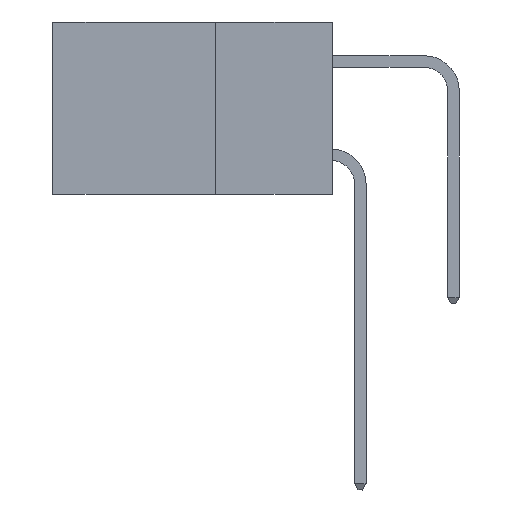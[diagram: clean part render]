
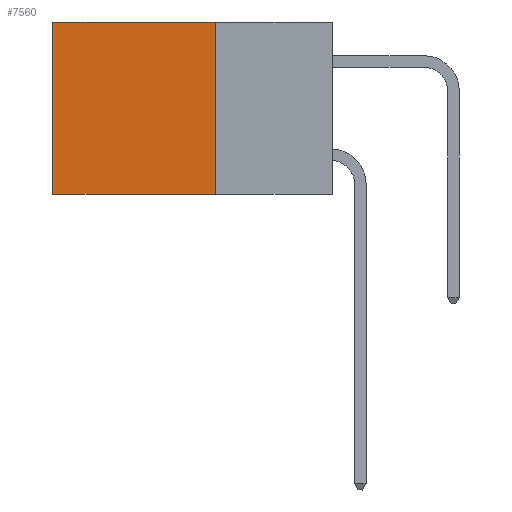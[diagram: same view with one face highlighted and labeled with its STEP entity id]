
A CAD part, left-side view. The second image highlights one B-rep face of the part: STEP entity #7560.
In plain terms, the highlighted planar face has unit normal (-1, 0, 0).
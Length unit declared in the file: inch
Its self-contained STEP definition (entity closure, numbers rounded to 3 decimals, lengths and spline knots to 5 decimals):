
#1771 = CARTESIAN_POINT ( 'NONE',  ( 0.298, 0.6, -0.37 ) ) ;
#1935 = VERTEX_POINT ( 'NONE', #1771 ) ;
#2220 = VERTEX_POINT ( 'NONE', #6281 ) ;
#3377 = VERTEX_POINT ( 'NONE', #13682 ) ;
#3509 = CARTESIAN_POINT ( 'NONE',  ( 0.298, 0.25, 0. ) ) ;
#3619 = PLANE ( 'NONE',  #9586 ) ;
#3799 = LINE ( 'NONE', #27480, #14347 ) ;
#5038 = CARTESIAN_POINT ( 'NONE',  ( 0.298, 0.25, -0.37 ) ) ;
#5067 = LINE ( 'NONE', #11138, #21648 ) ;
#6281 = CARTESIAN_POINT ( 'NONE',  ( 0.298, 0.25, 0. ) ) ;
#7109 = EDGE_CURVE ( 'NONE', #2220, #3377, #5067, .T. ) ;
#7560 = ADVANCED_FACE ( 'NONE', ( #19755 ), #3619, .F. ) ;
#7926 = DIRECTION ( 'NONE',  ( 0., 0., -1. ) ) ;
#9586 = AXIS2_PLACEMENT_3D ( 'NONE', #3509, #17624, #7926 ) ;
#11138 = CARTESIAN_POINT ( 'NONE',  ( 0.298, 0.25, 0. ) ) ;
#11330 = EDGE_CURVE ( 'NONE', #3377, #1935, #28013, .T. ) ;
#11387 = CARTESIAN_POINT ( 'NONE',  ( 0.298, 0.6, 0. ) ) ;
#13682 = CARTESIAN_POINT ( 'NONE',  ( 0.298, 0.25, -0.37 ) ) ;
#14172 = DIRECTION ( 'NONE',  ( 0., 1., 0. ) ) ;
#14347 = VECTOR ( 'NONE', #14172, 39.37008 ) ;
#15001 = VERTEX_POINT ( 'NONE', #24747 ) ;
#15142 = ORIENTED_EDGE ( 'NONE', *, *, #24478, .T. ) ;
#15784 = LINE ( 'NONE', #11387, #28147 ) ;
#16204 = ORIENTED_EDGE ( 'NONE', *, *, #16636, .T. ) ;
#16326 = ORIENTED_EDGE ( 'NONE', *, *, #7109, .F. ) ;
#16636 = EDGE_CURVE ( 'NONE', #2220, #15001, #3799, .T. ) ;
#17060 = DIRECTION ( 'NONE',  ( 0., 1., 0. ) ) ;
#17624 = DIRECTION ( 'NONE',  ( 1., 0., 0. ) ) ;
#19755 = FACE_OUTER_BOUND ( 'NONE', #23941, .T. ) ;
#20895 = VECTOR ( 'NONE', #17060, 39.37008 ) ;
#20936 = DIRECTION ( 'NONE',  ( 0., 0., -1. ) ) ;
#21648 = VECTOR ( 'NONE', #30053, 39.37008 ) ;
#23941 = EDGE_LOOP ( 'NONE', ( #15142, #26551, #16326, #16204 ) ) ;
#24478 = EDGE_CURVE ( 'NONE', #15001, #1935, #15784, .T. ) ;
#24747 = CARTESIAN_POINT ( 'NONE',  ( 0.298, 0.6, 0. ) ) ;
#26551 = ORIENTED_EDGE ( 'NONE', *, *, #11330, .F. ) ;
#27480 = CARTESIAN_POINT ( 'NONE',  ( 0.298, 0.25, 0. ) ) ;
#28013 = LINE ( 'NONE', #5038, #20895 ) ;
#28147 = VECTOR ( 'NONE', #20936, 39.37008 ) ;
#30053 = DIRECTION ( 'NONE',  ( 0., 0., -1. ) ) ;
